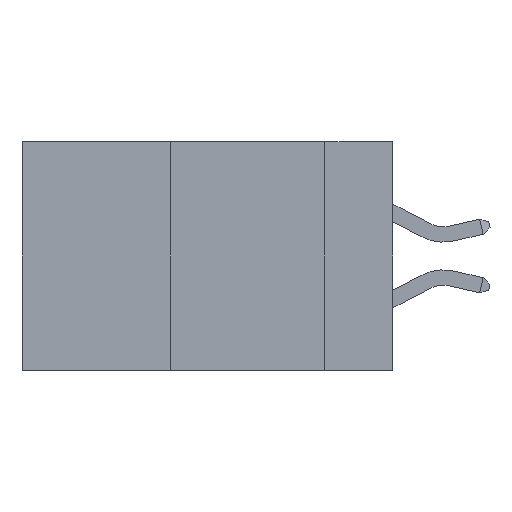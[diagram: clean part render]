
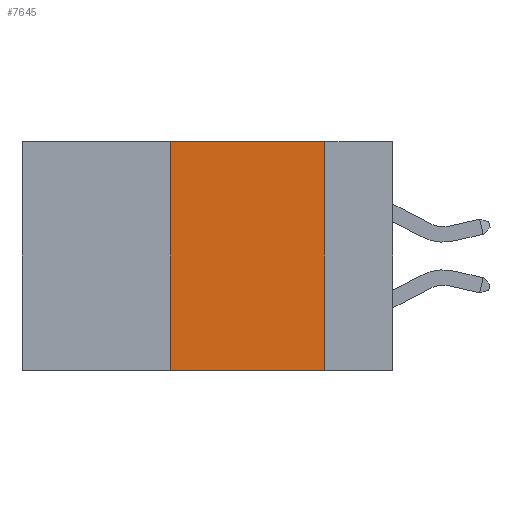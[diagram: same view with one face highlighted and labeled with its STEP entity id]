
A CAD part, left-side view. The second image highlights one B-rep face of the part: STEP entity #7645.
In plain terms, the highlighted planar face has unit normal (-1, 0, 0).
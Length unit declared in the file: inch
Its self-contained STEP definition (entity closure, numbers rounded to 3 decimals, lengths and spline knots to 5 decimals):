
#107 = VECTOR ( 'NONE', #5932, 39.37008 ) ;
#199 = VERTEX_POINT ( 'NONE', #7501 ) ;
#948 = VECTOR ( 'NONE', #8057, 39.37008 ) ;
#1080 = CARTESIAN_POINT ( 'NONE',  ( 0., 0.11, 0. ) ) ;
#1114 = VECTOR ( 'NONE', #2307, 39.37008 ) ;
#1144 = LINE ( 'NONE', #3613, #1273 ) ;
#1273 = VECTOR ( 'NONE', #2817, 39.37008 ) ;
#1422 = DIRECTION ( 'NONE',  ( 1., 0., 0. ) ) ;
#1944 = ORIENTED_EDGE ( 'NONE', *, *, #8136, .F. ) ;
#2022 = CARTESIAN_POINT ( 'NONE',  ( 0., 0.36, 0. ) ) ;
#2156 = DIRECTION ( 'NONE',  ( 0., 0., -1. ) ) ;
#2307 = DIRECTION ( 'NONE',  ( 0., -1., 0. ) ) ;
#2671 = LINE ( 'NONE', #3137, #1114 ) ;
#2817 = DIRECTION ( 'NONE',  ( 0., 0., -1. ) ) ;
#3109 = LINE ( 'NONE', #2022, #107 ) ;
#3137 = CARTESIAN_POINT ( 'NONE',  ( 0., 0.6, 0. ) ) ;
#3478 = CARTESIAN_POINT ( 'NONE',  ( 0., 0.11, -0.37 ) ) ;
#3613 = CARTESIAN_POINT ( 'NONE',  ( 0., 0.11, 0. ) ) ;
#3629 = VERTEX_POINT ( 'NONE', #9597 ) ;
#3769 = PLANE ( 'NONE',  #7679 ) ;
#3791 = EDGE_CURVE ( 'NONE', #5732, #4812, #1144, .T. ) ;
#4315 = FACE_OUTER_BOUND ( 'NONE', #7275, .T. ) ;
#4812 = VERTEX_POINT ( 'NONE', #3478 ) ;
#5281 = EDGE_CURVE ( 'NONE', #3629, #5732, #2671, .T. ) ;
#5296 = LINE ( 'NONE', #6518, #948 ) ;
#5732 = VERTEX_POINT ( 'NONE', #1080 ) ;
#5932 = DIRECTION ( 'NONE',  ( 0., 0., 1. ) ) ;
#6518 = CARTESIAN_POINT ( 'NONE',  ( 0., 0.6, -0.37 ) ) ;
#6771 = ORIENTED_EDGE ( 'NONE', *, *, #5281, .F. ) ;
#7275 = EDGE_LOOP ( 'NONE', ( #7527, #6771, #1944, #7498 ) ) ;
#7498 = ORIENTED_EDGE ( 'NONE', *, *, #7558, .T. ) ;
#7501 = CARTESIAN_POINT ( 'NONE',  ( 0., 0.36, -0.37 ) ) ;
#7527 = ORIENTED_EDGE ( 'NONE', *, *, #3791, .F. ) ;
#7558 = EDGE_CURVE ( 'NONE', #199, #4812, #5296, .T. ) ;
#7645 = ADVANCED_FACE ( 'NONE', ( #4315 ), #3769, .F. ) ;
#7679 = AXIS2_PLACEMENT_3D ( 'NONE', #9739, #1422, #2156 ) ;
#8057 = DIRECTION ( 'NONE',  ( 0., -1., 0. ) ) ;
#8136 = EDGE_CURVE ( 'NONE', #199, #3629, #3109, .T. ) ;
#9597 = CARTESIAN_POINT ( 'NONE',  ( 0., 0.36, 0. ) ) ;
#9739 = CARTESIAN_POINT ( 'NONE',  ( 0., 0.6, 0. ) ) ;
